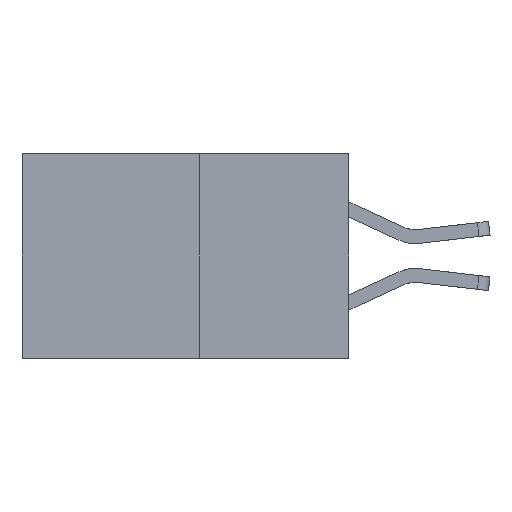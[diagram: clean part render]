
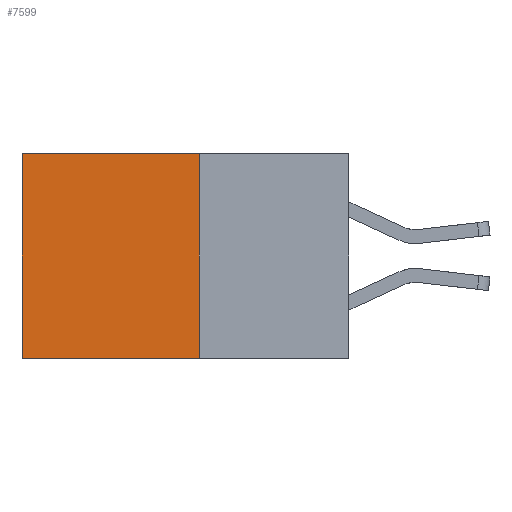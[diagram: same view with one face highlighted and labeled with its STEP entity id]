
A CAD part, left-side view. The second image highlights one B-rep face of the part: STEP entity #7599.
In plain terms, the highlighted planar face has unit normal (-1, 0, 0).
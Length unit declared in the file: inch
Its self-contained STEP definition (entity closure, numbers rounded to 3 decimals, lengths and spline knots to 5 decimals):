
#15 = EDGE_CURVE ( 'NONE', #4954, #607, #9634, .T. ) ;
#416 = ORIENTED_EDGE ( 'NONE', *, *, #15, .T. ) ;
#607 = VERTEX_POINT ( 'NONE', #2814 ) ;
#714 = VERTEX_POINT ( 'NONE', #3474 ) ;
#720 = LINE ( 'NONE', #8742, #2567 ) ;
#1017 = VECTOR ( 'NONE', #2477, 39.37008 ) ;
#1556 = EDGE_CURVE ( 'NONE', #714, #2432, #7134, .T. ) ;
#1819 = ORIENTED_EDGE ( 'NONE', *, *, #1556, .F. ) ;
#1943 = VECTOR ( 'NONE', #8264, 39.37008 ) ;
#2421 = DIRECTION ( 'NONE',  ( 0., 0., -1. ) ) ;
#2423 = EDGE_LOOP ( 'NONE', ( #8175, #1819, #2765, #416 ) ) ;
#2432 = VERTEX_POINT ( 'NONE', #7237 ) ;
#2477 = DIRECTION ( 'NONE',  ( 0., 1., 0. ) ) ;
#2567 = VECTOR ( 'NONE', #2421, 39.37008 ) ;
#2667 = EDGE_CURVE ( 'NONE', #4954, #714, #720, .T. ) ;
#2765 = ORIENTED_EDGE ( 'NONE', *, *, #2667, .F. ) ;
#2814 = CARTESIAN_POINT ( 'NONE',  ( 0.277, 0.59, 0. ) ) ;
#3474 = CARTESIAN_POINT ( 'NONE',  ( 0.277, 0.27, -0.37 ) ) ;
#4560 = VECTOR ( 'NONE', #6895, 39.37008 ) ;
#4824 = DIRECTION ( 'NONE',  ( 1., 0., 0. ) ) ;
#4875 = DIRECTION ( 'NONE',  ( 0., 0., -1. ) ) ;
#4954 = VERTEX_POINT ( 'NONE', #7593 ) ;
#5110 = CARTESIAN_POINT ( 'NONE',  ( 0.277, 0.27, -0.37 ) ) ;
#5135 = CARTESIAN_POINT ( 'NONE',  ( 0.277, 0.27, -0.37 ) ) ;
#5497 = PLANE ( 'NONE',  #7413 ) ;
#6895 = DIRECTION ( 'NONE',  ( 0., 0., -1. ) ) ;
#6920 = EDGE_CURVE ( 'NONE', #607, #2432, #8440, .T. ) ;
#6946 = CARTESIAN_POINT ( 'NONE',  ( 0.277, 0.59, -0.37 ) ) ;
#7134 = LINE ( 'NONE', #5135, #1017 ) ;
#7237 = CARTESIAN_POINT ( 'NONE',  ( 0.277, 0.59, -0.37 ) ) ;
#7413 = AXIS2_PLACEMENT_3D ( 'NONE', #5110, #4824, #4875 ) ;
#7593 = CARTESIAN_POINT ( 'NONE',  ( 0.277, 0.27, 0. ) ) ;
#7599 = ADVANCED_FACE ( 'NONE', ( #8982 ), #5497, .F. ) ;
#8175 = ORIENTED_EDGE ( 'NONE', *, *, #6920, .T. ) ;
#8264 = DIRECTION ( 'NONE',  ( 0., 1., 0. ) ) ;
#8440 = LINE ( 'NONE', #6946, #4560 ) ;
#8716 = CARTESIAN_POINT ( 'NONE',  ( 0.277, 0.27, 0. ) ) ;
#8742 = CARTESIAN_POINT ( 'NONE',  ( 0.277, 0.27, -0.37 ) ) ;
#8982 = FACE_OUTER_BOUND ( 'NONE', #2423, .T. ) ;
#9634 = LINE ( 'NONE', #8716, #1943 ) ;
